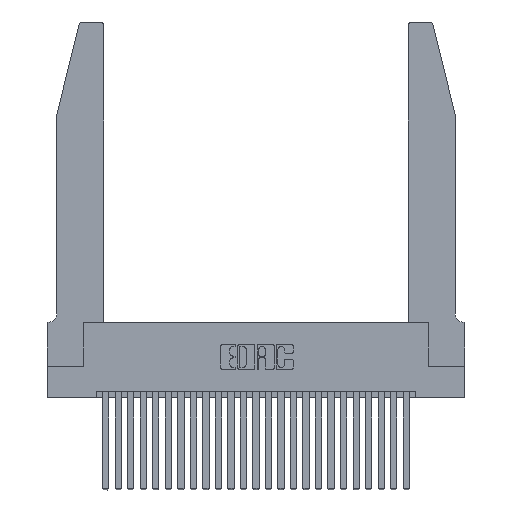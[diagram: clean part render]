
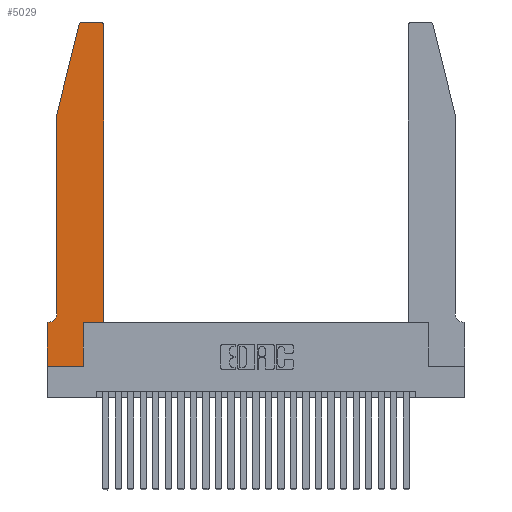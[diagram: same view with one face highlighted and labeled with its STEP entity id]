
A CAD part, top view. The second image highlights one B-rep face of the part: STEP entity #5029.
In plain terms, the highlighted planar face has unit normal (0, 0, 1).
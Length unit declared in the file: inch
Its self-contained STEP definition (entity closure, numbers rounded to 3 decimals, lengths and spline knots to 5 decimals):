
#4 = DIRECTION ( 'NONE',  ( 0., 1., 0. ) ) ;
#6 = ORIENTED_EDGE ( 'NONE', *, *, #6755, .T. ) ;
#123 = LINE ( 'NONE', #9850, #16758 ) ;
#286 = CARTESIAN_POINT ( 'NONE',  ( 0.0755, 0.35, 0.37 ) ) ;
#303 = VERTEX_POINT ( 'NONE', #16744 ) ;
#652 = CARTESIAN_POINT ( 'NONE',  ( 0.0055, 0.42, 0.37 ) ) ;
#789 = LINE ( 'NONE', #4959, #22520 ) ;
#795 = VERTEX_POINT ( 'NONE', #2744 ) ;
#1122 = LINE ( 'NONE', #12548, #20610 ) ;
#1156 = EDGE_CURVE ( 'NONE', #22718, #12164, #15746, .T. ) ;
#1669 = DIRECTION ( 'NONE',  ( 0., 0., 1. ) ) ;
#1704 = CARTESIAN_POINT ( 'NONE',  ( 0.4505, 0.35, 0.37 ) ) ;
#2133 = VERTEX_POINT ( 'NONE', #10025 ) ;
#2379 = CARTESIAN_POINT ( 'NONE',  ( 0.2605, 2.75, 0.37 ) ) ;
#2744 = CARTESIAN_POINT ( 'NONE',  ( 0., 0.35, 0.37 ) ) ;
#4441 = DIRECTION ( 'NONE',  ( -1., 0., 0. ) ) ;
#4575 = CIRCLE ( 'NONE', #18780, 0.03 ) ;
#4723 = CARTESIAN_POINT ( 'NONE',  ( 0.2865, 0.35, 0.37 ) ) ;
#4732 = VERTEX_POINT ( 'NONE', #25237 ) ;
#4959 = CARTESIAN_POINT ( 'NONE',  ( 0., 0., 0.37 ) ) ;
#5029 = ADVANCED_FACE ( 'NONE', ( #15742 ), #21773, .T. ) ;
#5325 = LINE ( 'NONE', #7379, #9444 ) ;
#5652 = DIRECTION ( 'NONE',  ( 1., 0., 0. ) ) ;
#6134 = AXIS2_PLACEMENT_3D ( 'NONE', #652, #22882, #17013 ) ;
#6743 = DIRECTION ( 'NONE',  ( 0., -1., 0. ) ) ;
#6755 = EDGE_CURVE ( 'NONE', #7858, #9331, #13393, .T. ) ;
#6864 = ORIENTED_EDGE ( 'NONE', *, *, #11884, .T. ) ;
#7379 = CARTESIAN_POINT ( 'NONE',  ( 0.0755, 2., 0.37 ) ) ;
#7504 = VERTEX_POINT ( 'NONE', #9150 ) ;
#7730 = DIRECTION ( 'NONE',  ( -0.239, -0.971, 0. ) ) ;
#7858 = VERTEX_POINT ( 'NONE', #10601 ) ;
#9150 = CARTESIAN_POINT ( 'NONE',  ( 0.4505, 0.35, 0.37 ) ) ;
#9331 = VERTEX_POINT ( 'NONE', #10960 ) ;
#9444 = VECTOR ( 'NONE', #11371, 39.37008 ) ;
#9483 = ORIENTED_EDGE ( 'NONE', *, *, #12677, .T. ) ;
#9645 = CARTESIAN_POINT ( 'NONE',  ( 0.2865, 0.35, 0.37 ) ) ;
#9850 = CARTESIAN_POINT ( 'NONE',  ( 0.0755, 2., 0.37 ) ) ;
#9885 = ORIENTED_EDGE ( 'NONE', *, *, #1156, .T. ) ;
#10025 = CARTESIAN_POINT ( 'NONE',  ( 0.25487, 2.72718, 0.37 ) ) ;
#10048 = CARTESIAN_POINT ( 'NONE',  ( 0.0755, 0.42, 0.37 ) ) ;
#10256 = EDGE_CURVE ( 'NONE', #795, #303, #789, .T. ) ;
#10479 = CARTESIAN_POINT ( 'NONE',  ( 0.4505, 0.35, 0.37 ) ) ;
#10601 = CARTESIAN_POINT ( 'NONE',  ( 0.4505, 2.72, 0.37 ) ) ;
#10960 = CARTESIAN_POINT ( 'NONE',  ( 0.4205, 2.75, 0.37 ) ) ;
#11371 = DIRECTION ( 'NONE',  ( 0., -1., 0. ) ) ;
#11598 = EDGE_CURVE ( 'NONE', #19754, #4732, #16835, .T. ) ;
#11685 = DIRECTION ( 'NONE',  ( 0., 1., 0. ) ) ;
#11884 = EDGE_CURVE ( 'NONE', #13562, #19754, #5325, .T. ) ;
#12164 = VERTEX_POINT ( 'NONE', #4723 ) ;
#12341 = AXIS2_PLACEMENT_3D ( 'NONE', #25876, #25965, #20919 ) ;
#12522 = DIRECTION ( 'NONE',  ( -1., 0., 0. ) ) ;
#12548 = CARTESIAN_POINT ( 'NONE',  ( 0., 0., 0.37 ) ) ;
#12677 = EDGE_CURVE ( 'NONE', #2133, #13562, #123, .T. ) ;
#13127 = LINE ( 'NONE', #2379, #24321 ) ;
#13393 = CIRCLE ( 'NONE', #12341, 0.03 ) ;
#13562 = VERTEX_POINT ( 'NONE', #17043 ) ;
#13866 = CARTESIAN_POINT ( 'NONE',  ( 0.284, 2.75, 0.37 ) ) ;
#13870 = CARTESIAN_POINT ( 'NONE',  ( 0.284, 2.72, 0.37 ) ) ;
#14217 = EDGE_CURVE ( 'NONE', #9331, #24895, #13127, .T. ) ;
#15101 = VECTOR ( 'NONE', #11685, 39.37008 ) ;
#15739 = LINE ( 'NONE', #1704, #21809 ) ;
#15742 = FACE_OUTER_BOUND ( 'NONE', #25559, .T. ) ;
#15746 = LINE ( 'NONE', #9645, #15101 ) ;
#15942 = DIRECTION ( 'NONE',  ( 1., 0., 0. ) ) ;
#16074 = DIRECTION ( 'NONE',  ( 1., 0., 0. ) ) ;
#16744 = CARTESIAN_POINT ( 'NONE',  ( 0., 0., 0.37 ) ) ;
#16758 = VECTOR ( 'NONE', #7730, 39.37008 ) ;
#16835 = CIRCLE ( 'NONE', #6134, 0.07 ) ;
#17013 = DIRECTION ( 'NONE',  ( -1., 0., 0. ) ) ;
#17016 = LINE ( 'NONE', #286, #17659 ) ;
#17043 = CARTESIAN_POINT ( 'NONE',  ( 0.0755, 2., 0.37 ) ) ;
#17180 = LINE ( 'NONE', #10479, #23865 ) ;
#17384 = ORIENTED_EDGE ( 'NONE', *, *, #17707, .T. ) ;
#17470 = ORIENTED_EDGE ( 'NONE', *, *, #24535, .T. ) ;
#17659 = VECTOR ( 'NONE', #4441, 39.37008 ) ;
#17707 = EDGE_CURVE ( 'NONE', #7504, #7858, #17180, .T. ) ;
#17873 = CARTESIAN_POINT ( 'NONE',  ( 0., 0.35, 0.37 ) ) ;
#18780 = AXIS2_PLACEMENT_3D ( 'NONE', #13870, #1669, #15942 ) ;
#18980 = CARTESIAN_POINT ( 'NONE',  ( 0.2865, 0., 0.37 ) ) ;
#19158 = EDGE_CURVE ( 'NONE', #12164, #7504, #15739, .T. ) ;
#19481 = ORIENTED_EDGE ( 'NONE', *, *, #10256, .T. ) ;
#19754 = VERTEX_POINT ( 'NONE', #10048 ) ;
#19781 = EDGE_CURVE ( 'NONE', #24895, #2133, #4575, .T. ) ;
#19902 = EDGE_CURVE ( 'NONE', #4732, #795, #17016, .T. ) ;
#20610 = VECTOR ( 'NONE', #25064, 39.37008 ) ;
#20919 = DIRECTION ( 'NONE',  ( 1., 0., 0. ) ) ;
#20990 = ORIENTED_EDGE ( 'NONE', *, *, #19902, .T. ) ;
#21316 = ORIENTED_EDGE ( 'NONE', *, *, #19781, .T. ) ;
#21586 = DIRECTION ( 'NONE',  ( 0., 0., 1. ) ) ;
#21655 = ORIENTED_EDGE ( 'NONE', *, *, #11598, .T. ) ;
#21773 = PLANE ( 'NONE',  #25498 ) ;
#21809 = VECTOR ( 'NONE', #16074, 39.37008 ) ;
#22520 = VECTOR ( 'NONE', #6743, 39.37008 ) ;
#22718 = VERTEX_POINT ( 'NONE', #18980 ) ;
#22882 = DIRECTION ( 'NONE',  ( 0., 0., -1. ) ) ;
#23154 = ORIENTED_EDGE ( 'NONE', *, *, #14217, .T. ) ;
#23571 = ORIENTED_EDGE ( 'NONE', *, *, #19158, .T. ) ;
#23865 = VECTOR ( 'NONE', #4, 39.37008 ) ;
#24321 = VECTOR ( 'NONE', #12522, 39.37008 ) ;
#24535 = EDGE_CURVE ( 'NONE', #303, #22718, #1122, .T. ) ;
#24895 = VERTEX_POINT ( 'NONE', #13866 ) ;
#25064 = DIRECTION ( 'NONE',  ( 1., 0., 0. ) ) ;
#25237 = CARTESIAN_POINT ( 'NONE',  ( 0.0055, 0.35, 0.37 ) ) ;
#25498 = AXIS2_PLACEMENT_3D ( 'NONE', #17873, #21586, #5652 ) ;
#25559 = EDGE_LOOP ( 'NONE', ( #23154, #21316, #9483, #6864, #21655, #20990, #19481, #17470, #9885, #23571, #17384, #6 ) ) ;
#25876 = CARTESIAN_POINT ( 'NONE',  ( 0.4205, 2.72, 0.37 ) ) ;
#25965 = DIRECTION ( 'NONE',  ( 0., 0., 1. ) ) ;
